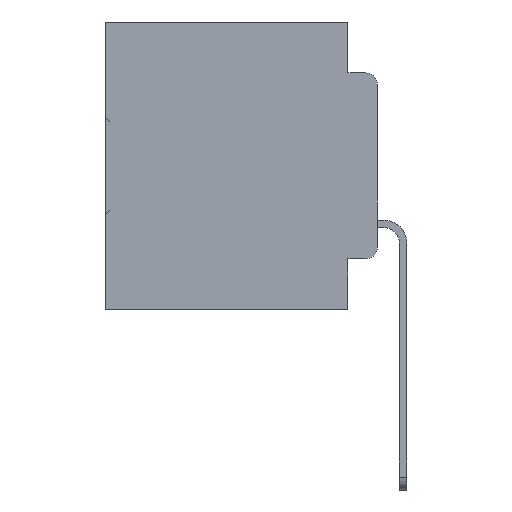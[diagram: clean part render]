
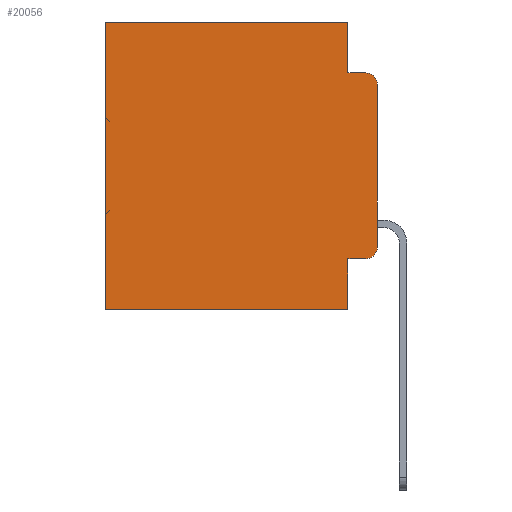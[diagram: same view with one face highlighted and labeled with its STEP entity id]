
A CAD part, left-side view. The second image highlights one B-rep face of the part: STEP entity #20056.
In plain terms, the highlighted planar face has unit normal (-1, 0, 0).
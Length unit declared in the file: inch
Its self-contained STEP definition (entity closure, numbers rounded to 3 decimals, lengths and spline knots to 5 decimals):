
#396 = DIRECTION ( 'NONE',  ( 0., 0., -1. ) ) ;
#451 = VECTOR ( 'NONE', #36055, 39.37008 ) ;
#574 = EDGE_CURVE ( 'NONE', #7575, #26375, #4753, .T. ) ;
#820 = EDGE_CURVE ( 'NONE', #28028, #28576, #35163, .T. ) ;
#1082 = CARTESIAN_POINT ( 'NONE',  ( 0.298, 0.051, 0. ) ) ;
#1314 = DIRECTION ( 'NONE',  ( 0., 0., -1. ) ) ;
#1408 = CARTESIAN_POINT ( 'NONE',  ( 0.298, 0., 0. ) ) ;
#2126 = LINE ( 'NONE', #3541, #16979 ) ;
#2942 = EDGE_CURVE ( 'NONE', #30930, #28028, #37220, .T. ) ;
#2982 = VERTEX_POINT ( 'NONE', #4475 ) ;
#3397 = VERTEX_POINT ( 'NONE', #6277 ) ;
#3475 = LINE ( 'NONE', #28745, #25911 ) ;
#3541 = CARTESIAN_POINT ( 'NONE',  ( 0.298, 0.473, 0. ) ) ;
#3755 = DIRECTION ( 'NONE',  ( -1., 0., 0. ) ) ;
#4060 = ORIENTED_EDGE ( 'NONE', *, *, #4217, .F. ) ;
#4136 = VECTOR ( 'NONE', #19144, 39.37008 ) ;
#4149 = VECTOR ( 'NONE', #15371, 39.37008 ) ;
#4217 = EDGE_CURVE ( 'NONE', #34108, #26375, #16028, .T. ) ;
#4475 = CARTESIAN_POINT ( 'NONE',  ( 0.298, 0.473, 0. ) ) ;
#4753 = CIRCLE ( 'NONE', #37300, 0.02 ) ;
#4993 = LINE ( 'NONE', #33152, #9162 ) ;
#6277 = CARTESIAN_POINT ( 'NONE',  ( 0.298, 0.051, 0. ) ) ;
#6420 = DIRECTION ( 'NONE',  ( 0., 0., -1. ) ) ;
#6452 = DIRECTION ( 'NONE',  ( -1., 0., 0. ) ) ;
#7575 = VERTEX_POINT ( 'NONE', #31475 ) ;
#7804 = ORIENTED_EDGE ( 'NONE', *, *, #15900, .F. ) ;
#7907 = DIRECTION ( 'NONE',  ( 0., -1., 0. ) ) ;
#8034 = CARTESIAN_POINT ( 'NONE',  ( 0.298, 0.02, -0.1085 ) ) ;
#9162 = VECTOR ( 'NONE', #9977, 39.37008 ) ;
#9422 = EDGE_LOOP ( 'NONE', ( #7804, #21259, #4060, #23527, #29814, #9888, #11164, #29179, #23981, #20785 ) ) ;
#9888 = ORIENTED_EDGE ( 'NONE', *, *, #14911, .T. ) ;
#9977 = DIRECTION ( 'NONE',  ( 0., 1., 0. ) ) ;
#11164 = ORIENTED_EDGE ( 'NONE', *, *, #18083, .F. ) ;
#12963 = EDGE_CURVE ( 'NONE', #30930, #30667, #25649, .T. ) ;
#13896 = CARTESIAN_POINT ( 'NONE',  ( 0.298, 0.051, -0.0885 ) ) ;
#14911 = EDGE_CURVE ( 'NONE', #2982, #29644, #2126, .T. ) ;
#15371 = DIRECTION ( 'NONE',  ( 0., 0., -1. ) ) ;
#15497 = CARTESIAN_POINT ( 'NONE',  ( 0.298, 0.051, 0. ) ) ;
#15900 = EDGE_CURVE ( 'NONE', #7575, #28576, #3475, .T. ) ;
#15993 = CARTESIAN_POINT ( 'NONE',  ( 0.298, 0.051, -0.4115 ) ) ;
#16028 = LINE ( 'NONE', #13896, #22785 ) ;
#16146 = CARTESIAN_POINT ( 'NONE',  ( 0.298, 0.051, -0.5 ) ) ;
#16193 = CARTESIAN_POINT ( 'NONE',  ( 0.298, 0.02, -0.0885 ) ) ;
#16837 = EDGE_CURVE ( 'NONE', #3397, #34108, #17265, .T. ) ;
#16979 = VECTOR ( 'NONE', #396, 39.37008 ) ;
#17239 = CARTESIAN_POINT ( 'NONE',  ( 0.298, 0.051, -0.0885 ) ) ;
#17265 = LINE ( 'NONE', #1082, #451 ) ;
#17364 = CARTESIAN_POINT ( 'NONE',  ( 0.298, 0.051, -0.4115 ) ) ;
#17615 = DIRECTION ( 'NONE',  ( 1., 0., 0. ) ) ;
#18083 = EDGE_CURVE ( 'NONE', #30667, #29644, #4993, .T. ) ;
#19144 = DIRECTION ( 'NONE',  ( 0., 1., 0. ) ) ;
#20056 = ADVANCED_FACE ( 'NONE', ( #24937 ), #26191, .F. ) ;
#20785 = ORIENTED_EDGE ( 'NONE', *, *, #820, .T. ) ;
#21088 = VECTOR ( 'NONE', #27571, 39.37008 ) ;
#21259 = ORIENTED_EDGE ( 'NONE', *, *, #574, .T. ) ;
#22785 = VECTOR ( 'NONE', #7907, 39.37008 ) ;
#22966 = DIRECTION ( 'NONE',  ( 0., 0., -1. ) ) ;
#23527 = ORIENTED_EDGE ( 'NONE', *, *, #16837, .F. ) ;
#23981 = ORIENTED_EDGE ( 'NONE', *, *, #2942, .T. ) ;
#24937 = FACE_OUTER_BOUND ( 'NONE', #9422, .T. ) ;
#25649 = LINE ( 'NONE', #15497, #4149 ) ;
#25911 = VECTOR ( 'NONE', #22966, 39.37008 ) ;
#26191 = PLANE ( 'NONE',  #34719 ) ;
#26375 = VERTEX_POINT ( 'NONE', #16193 ) ;
#27256 = CARTESIAN_POINT ( 'NONE',  ( 0.298, 0., -0.3915 ) ) ;
#27436 = LINE ( 'NONE', #1408, #4136 ) ;
#27571 = DIRECTION ( 'NONE',  ( 0., -1., 0. ) ) ;
#28028 = VERTEX_POINT ( 'NONE', #33459 ) ;
#28576 = VERTEX_POINT ( 'NONE', #27256 ) ;
#28745 = CARTESIAN_POINT ( 'NONE',  ( 0.298, 0., 0. ) ) ;
#28942 = AXIS2_PLACEMENT_3D ( 'NONE', #36935, #6452, #6420 ) ;
#29179 = ORIENTED_EDGE ( 'NONE', *, *, #12963, .F. ) ;
#29644 = VERTEX_POINT ( 'NONE', #35554 ) ;
#29814 = ORIENTED_EDGE ( 'NONE', *, *, #30691, .T. ) ;
#30667 = VERTEX_POINT ( 'NONE', #16146 ) ;
#30691 = EDGE_CURVE ( 'NONE', #3397, #2982, #27436, .T. ) ;
#30930 = VERTEX_POINT ( 'NONE', #17364 ) ;
#31475 = CARTESIAN_POINT ( 'NONE',  ( 0.298, 0., -0.1085 ) ) ;
#33152 = CARTESIAN_POINT ( 'NONE',  ( 0.298, 0., -0.5 ) ) ;
#33459 = CARTESIAN_POINT ( 'NONE',  ( 0.298, 0.02, -0.4115 ) ) ;
#34108 = VERTEX_POINT ( 'NONE', #17239 ) ;
#34719 = AXIS2_PLACEMENT_3D ( 'NONE', #34832, #17615, #37676 ) ;
#34832 = CARTESIAN_POINT ( 'NONE',  ( 0.298, 0., 0. ) ) ;
#35163 = CIRCLE ( 'NONE', #28942, 0.02 ) ;
#35554 = CARTESIAN_POINT ( 'NONE',  ( 0.298, 0.473, -0.5 ) ) ;
#36055 = DIRECTION ( 'NONE',  ( 0., 0., -1. ) ) ;
#36935 = CARTESIAN_POINT ( 'NONE',  ( 0.298, 0.02, -0.3915 ) ) ;
#37220 = LINE ( 'NONE', #15993, #21088 ) ;
#37300 = AXIS2_PLACEMENT_3D ( 'NONE', #8034, #3755, #1314 ) ;
#37676 = DIRECTION ( 'NONE',  ( 0., 0., -1. ) ) ;
